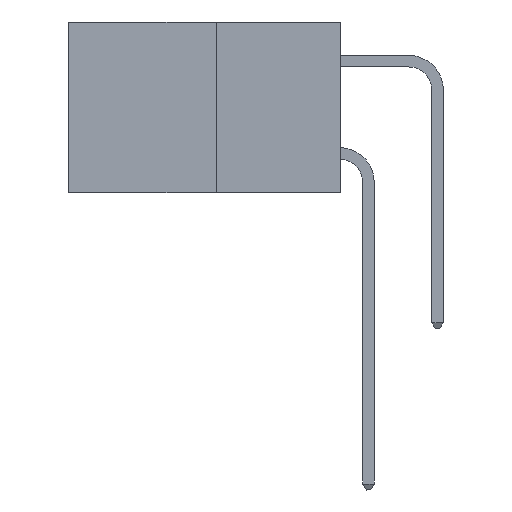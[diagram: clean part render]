
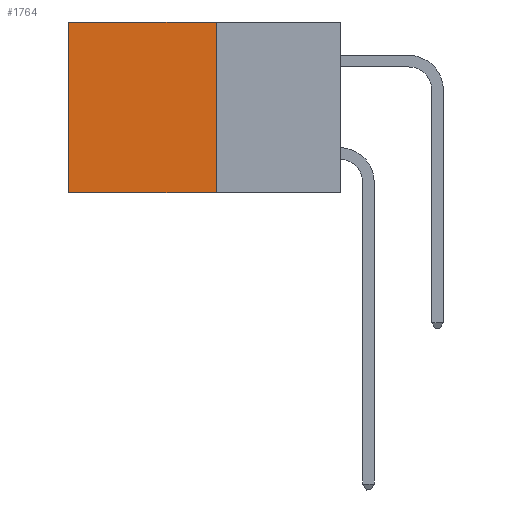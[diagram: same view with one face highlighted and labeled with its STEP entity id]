
A CAD part, left-side view. The second image highlights one B-rep face of the part: STEP entity #1764.
In plain terms, the highlighted planar face has unit normal (-1, 0, 0).
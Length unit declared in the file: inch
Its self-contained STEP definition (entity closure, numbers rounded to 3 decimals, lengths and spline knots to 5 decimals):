
#500 = CARTESIAN_POINT ( 'NONE',  ( 0.277, 0.27, -0.37 ) ) ;
#682 = VERTEX_POINT ( 'NONE', #6305 ) ;
#751 = LINE ( 'NONE', #3169, #3035 ) ;
#790 = EDGE_LOOP ( 'NONE', ( #10494, #6014, #10536, #7386 ) ) ;
#823 = EDGE_CURVE ( 'NONE', #8197, #8338, #4594, .T. ) ;
#1764 = ADVANCED_FACE ( 'NONE', ( #2210 ), #3559, .F. ) ;
#2134 = CARTESIAN_POINT ( 'NONE',  ( 0.277, 0.27, 0. ) ) ;
#2206 = AXIS2_PLACEMENT_3D ( 'NONE', #8853, #9532, #2754 ) ;
#2210 = FACE_OUTER_BOUND ( 'NONE', #790, .T. ) ;
#2754 = DIRECTION ( 'NONE',  ( 0., 0., -1. ) ) ;
#3035 = VECTOR ( 'NONE', #10132, 39.37008 ) ;
#3169 = CARTESIAN_POINT ( 'NONE',  ( 0.277, 0.59, -0.37 ) ) ;
#3559 = PLANE ( 'NONE',  #2206 ) ;
#3788 = CARTESIAN_POINT ( 'NONE',  ( 0.277, 0.27, 0. ) ) ;
#4016 = VECTOR ( 'NONE', #6987, 39.37008 ) ;
#4594 = LINE ( 'NONE', #5247, #8683 ) ;
#5189 = VECTOR ( 'NONE', #5873, 39.37008 ) ;
#5247 = CARTESIAN_POINT ( 'NONE',  ( 0.277, 0.27, -0.37 ) ) ;
#5873 = DIRECTION ( 'NONE',  ( 0., 1., 0. ) ) ;
#6014 = ORIENTED_EDGE ( 'NONE', *, *, #10340, .F. ) ;
#6114 = DIRECTION ( 'NONE',  ( 0., 0., -1. ) ) ;
#6178 = LINE ( 'NONE', #500, #4016 ) ;
#6205 = VERTEX_POINT ( 'NONE', #10853 ) ;
#6305 = CARTESIAN_POINT ( 'NONE',  ( 0.277, 0.59, -0.37 ) ) ;
#6987 = DIRECTION ( 'NONE',  ( 0., 1., 0. ) ) ;
#7386 = ORIENTED_EDGE ( 'NONE', *, *, #8987, .T. ) ;
#7488 = LINE ( 'NONE', #2134, #5189 ) ;
#7571 = CARTESIAN_POINT ( 'NONE',  ( 0.277, 0.27, -0.37 ) ) ;
#8197 = VERTEX_POINT ( 'NONE', #3788 ) ;
#8338 = VERTEX_POINT ( 'NONE', #7571 ) ;
#8683 = VECTOR ( 'NONE', #6114, 39.37008 ) ;
#8853 = CARTESIAN_POINT ( 'NONE',  ( 0.277, 0.27, -0.37 ) ) ;
#8987 = EDGE_CURVE ( 'NONE', #8197, #6205, #7488, .T. ) ;
#9532 = DIRECTION ( 'NONE',  ( 1., 0., 0. ) ) ;
#10132 = DIRECTION ( 'NONE',  ( 0., 0., -1. ) ) ;
#10340 = EDGE_CURVE ( 'NONE', #8338, #682, #6178, .T. ) ;
#10494 = ORIENTED_EDGE ( 'NONE', *, *, #11231, .T. ) ;
#10536 = ORIENTED_EDGE ( 'NONE', *, *, #823, .F. ) ;
#10853 = CARTESIAN_POINT ( 'NONE',  ( 0.277, 0.59, 0. ) ) ;
#11231 = EDGE_CURVE ( 'NONE', #6205, #682, #751, .T. ) ;
